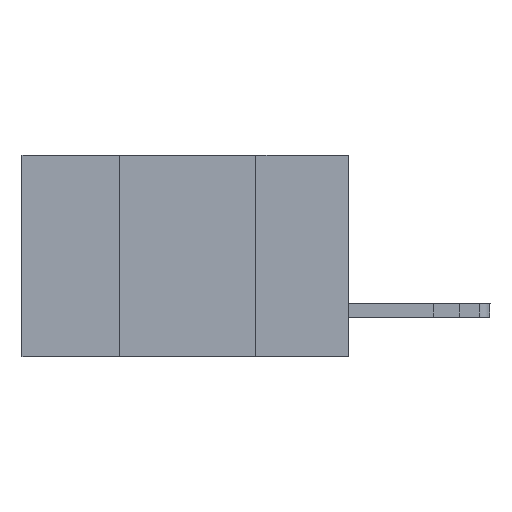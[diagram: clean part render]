
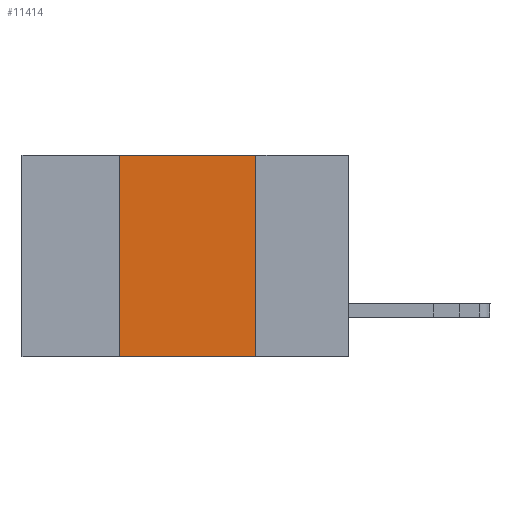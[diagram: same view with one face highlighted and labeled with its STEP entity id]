
A CAD part, left-side view. The second image highlights one B-rep face of the part: STEP entity #11414.
In plain terms, the highlighted planar face has unit normal (-1, 0, 0).
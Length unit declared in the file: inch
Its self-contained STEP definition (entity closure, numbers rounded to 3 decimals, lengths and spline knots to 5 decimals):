
#907 = CARTESIAN_POINT ( 'NONE',  ( 0., 0.17, 0. ) ) ;
#1317 = VERTEX_POINT ( 'NONE', #7757 ) ;
#2057 = LINE ( 'NONE', #18221, #6550 ) ;
#2076 = DIRECTION ( 'NONE',  ( 0., 0., -1. ) ) ;
#2116 = CARTESIAN_POINT ( 'NONE',  ( 0., 0.42, -0.37 ) ) ;
#2424 = PLANE ( 'NONE',  #8790 ) ;
#2747 = EDGE_CURVE ( 'NONE', #1317, #16781, #16633, .T. ) ;
#3023 = CARTESIAN_POINT ( 'NONE',  ( 0., 0.6, 0. ) ) ;
#3253 = DIRECTION ( 'NONE',  ( 0., -1., 0. ) ) ;
#3459 = LINE ( 'NONE', #6414, #16710 ) ;
#3797 = VECTOR ( 'NONE', #6080, 39.37008 ) ;
#4592 = EDGE_CURVE ( 'NONE', #16781, #12029, #15669, .T. ) ;
#4637 = CARTESIAN_POINT ( 'NONE',  ( 0., 0.17, -0.37 ) ) ;
#5277 = FACE_OUTER_BOUND ( 'NONE', #15062, .T. ) ;
#6080 = DIRECTION ( 'NONE',  ( 0., -1., 0. ) ) ;
#6414 = CARTESIAN_POINT ( 'NONE',  ( 0., 0.42, 0. ) ) ;
#6550 = VECTOR ( 'NONE', #3253, 39.37008 ) ;
#7757 = CARTESIAN_POINT ( 'NONE',  ( 0., 0.42, 0. ) ) ;
#8790 = AXIS2_PLACEMENT_3D ( 'NONE', #11356, #11548, #16419 ) ;
#9501 = CARTESIAN_POINT ( 'NONE',  ( 0., 0.17, 0. ) ) ;
#10706 = EDGE_CURVE ( 'NONE', #11104, #1317, #3459, .T. ) ;
#11104 = VERTEX_POINT ( 'NONE', #2116 ) ;
#11356 = CARTESIAN_POINT ( 'NONE',  ( 0., 0.6, 0. ) ) ;
#11414 = ADVANCED_FACE ( 'NONE', ( #5277 ), #2424, .F. ) ;
#11548 = DIRECTION ( 'NONE',  ( 1., 0., 0. ) ) ;
#12029 = VERTEX_POINT ( 'NONE', #4637 ) ;
#12761 = ORIENTED_EDGE ( 'NONE', *, *, #4592, .F. ) ;
#15062 = EDGE_LOOP ( 'NONE', ( #12761, #18110, #16146, #16472 ) ) ;
#15669 = LINE ( 'NONE', #9501, #19272 ) ;
#16146 = ORIENTED_EDGE ( 'NONE', *, *, #10706, .F. ) ;
#16419 = DIRECTION ( 'NONE',  ( 0., 0., -1. ) ) ;
#16472 = ORIENTED_EDGE ( 'NONE', *, *, #17066, .T. ) ;
#16633 = LINE ( 'NONE', #3023, #3797 ) ;
#16710 = VECTOR ( 'NONE', #16856, 39.37008 ) ;
#16781 = VERTEX_POINT ( 'NONE', #907 ) ;
#16856 = DIRECTION ( 'NONE',  ( 0., 0., 1. ) ) ;
#17066 = EDGE_CURVE ( 'NONE', #11104, #12029, #2057, .T. ) ;
#18110 = ORIENTED_EDGE ( 'NONE', *, *, #2747, .F. ) ;
#18221 = CARTESIAN_POINT ( 'NONE',  ( 0., 0.6, -0.37 ) ) ;
#19272 = VECTOR ( 'NONE', #2076, 39.37008 ) ;
